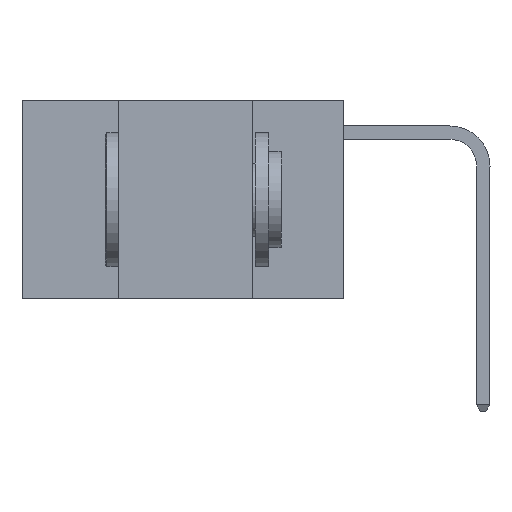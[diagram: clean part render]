
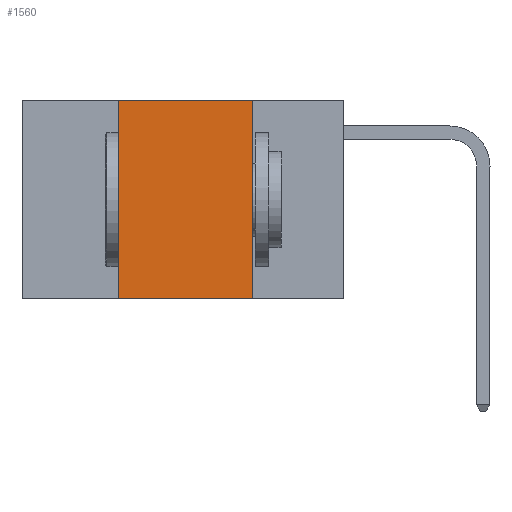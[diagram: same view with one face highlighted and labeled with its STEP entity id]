
A CAD part, left-side view. The second image highlights one B-rep face of the part: STEP entity #1560.
In plain terms, the highlighted planar face has unit normal (-1, 0, 0).
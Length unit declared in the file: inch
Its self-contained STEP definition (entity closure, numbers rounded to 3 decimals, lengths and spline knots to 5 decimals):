
#434 = VECTOR ( 'NONE', #9250, 39.37008 ) ;
#980 = AXIS2_PLACEMENT_3D ( 'NONE', #10755, #9630, #9563 ) ;
#1126 = ORIENTED_EDGE ( 'NONE', *, *, #4677, .F. ) ;
#1560 = ADVANCED_FACE ( 'NONE', ( #13308 ), #10018, .F. ) ;
#2752 = VERTEX_POINT ( 'NONE', #12721 ) ;
#2892 = EDGE_CURVE ( 'NONE', #11597, #4199, #5872, .T. ) ;
#2969 = ORIENTED_EDGE ( 'NONE', *, *, #14270, .F. ) ;
#3498 = EDGE_LOOP ( 'NONE', ( #1126, #2969, #13201, #5300 ) ) ;
#4199 = VERTEX_POINT ( 'NONE', #10665 ) ;
#4677 = EDGE_CURVE ( 'NONE', #2752, #15116, #16339, .T. ) ;
#4861 = LINE ( 'NONE', #7296, #15020 ) ;
#5300 = ORIENTED_EDGE ( 'NONE', *, *, #14782, .T. ) ;
#5872 = LINE ( 'NONE', #6097, #16405 ) ;
#6097 = CARTESIAN_POINT ( 'NONE',  ( 0., 0.42, 0. ) ) ;
#6171 = DIRECTION ( 'NONE',  ( 0., 0., 1. ) ) ;
#7296 = CARTESIAN_POINT ( 'NONE',  ( 0., 0.6, 0. ) ) ;
#8667 = DIRECTION ( 'NONE',  ( 0., -1., 0. ) ) ;
#8967 = VECTOR ( 'NONE', #14254, 39.37008 ) ;
#9250 = DIRECTION ( 'NONE',  ( 0., -1., 0. ) ) ;
#9563 = DIRECTION ( 'NONE',  ( 0., 0., -1. ) ) ;
#9630 = DIRECTION ( 'NONE',  ( 1., 0., 0. ) ) ;
#9714 = CARTESIAN_POINT ( 'NONE',  ( 0., 0.42, -0.37 ) ) ;
#10018 = PLANE ( 'NONE',  #980 ) ;
#10665 = CARTESIAN_POINT ( 'NONE',  ( 0., 0.42, 0. ) ) ;
#10755 = CARTESIAN_POINT ( 'NONE',  ( 0., 0.6, 0. ) ) ;
#11151 = LINE ( 'NONE', #11860, #434 ) ;
#11597 = VERTEX_POINT ( 'NONE', #9714 ) ;
#11860 = CARTESIAN_POINT ( 'NONE',  ( 0., 0.6, -0.37 ) ) ;
#12721 = CARTESIAN_POINT ( 'NONE',  ( 0., 0.17, 0. ) ) ;
#13201 = ORIENTED_EDGE ( 'NONE', *, *, #2892, .F. ) ;
#13308 = FACE_OUTER_BOUND ( 'NONE', #3498, .T. ) ;
#13832 = CARTESIAN_POINT ( 'NONE',  ( 0., 0.17, -0.37 ) ) ;
#14251 = CARTESIAN_POINT ( 'NONE',  ( 0., 0.17, 0. ) ) ;
#14254 = DIRECTION ( 'NONE',  ( 0., 0., -1. ) ) ;
#14270 = EDGE_CURVE ( 'NONE', #4199, #2752, #4861, .T. ) ;
#14782 = EDGE_CURVE ( 'NONE', #11597, #15116, #11151, .T. ) ;
#15020 = VECTOR ( 'NONE', #8667, 39.37008 ) ;
#15116 = VERTEX_POINT ( 'NONE', #13832 ) ;
#16339 = LINE ( 'NONE', #14251, #8967 ) ;
#16405 = VECTOR ( 'NONE', #6171, 39.37008 ) ;
